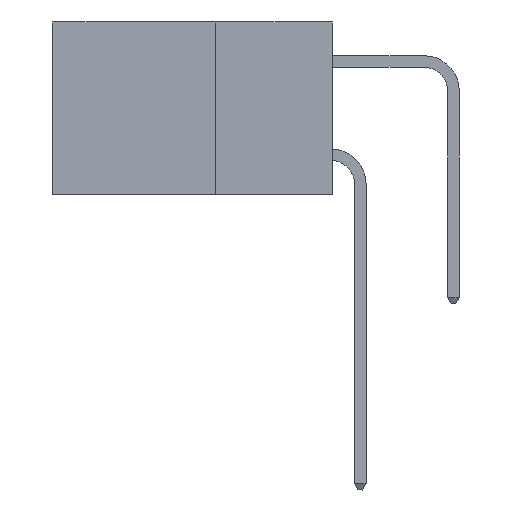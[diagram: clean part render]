
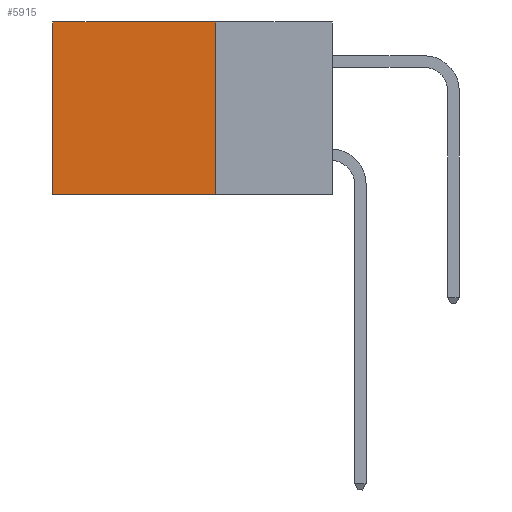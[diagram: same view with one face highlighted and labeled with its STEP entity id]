
A CAD part, left-side view. The second image highlights one B-rep face of the part: STEP entity #5915.
In plain terms, the highlighted planar face has unit normal (-1, 0, 0).
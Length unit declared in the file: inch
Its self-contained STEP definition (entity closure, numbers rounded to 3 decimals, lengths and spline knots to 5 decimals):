
#588 = EDGE_CURVE ( 'NONE', #13878, #1137, #4274, .T. ) ;
#701 = CARTESIAN_POINT ( 'NONE',  ( 0.298, 0.6, 0. ) ) ;
#1094 = EDGE_CURVE ( 'NONE', #13674, #3250, #10222, .T. ) ;
#1137 = VERTEX_POINT ( 'NONE', #9977 ) ;
#1223 = CARTESIAN_POINT ( 'NONE',  ( 0.298, 0.25, 0. ) ) ;
#1358 = DIRECTION ( 'NONE',  ( 0., 1., 0. ) ) ;
#1468 = ORIENTED_EDGE ( 'NONE', *, *, #588, .F. ) ;
#2970 = LINE ( 'NONE', #6909, #15835 ) ;
#3250 = VERTEX_POINT ( 'NONE', #701 ) ;
#3386 = ORIENTED_EDGE ( 'NONE', *, *, #10415, .F. ) ;
#4274 = LINE ( 'NONE', #13102, #8049 ) ;
#4414 = DIRECTION ( 'NONE',  ( 0., 0., -1. ) ) ;
#5915 = ADVANCED_FACE ( 'NONE', ( #8065 ), #13463, .F. ) ;
#5935 = EDGE_CURVE ( 'NONE', #3250, #1137, #11028, .T. ) ;
#6835 = VECTOR ( 'NONE', #1358, 39.37008 ) ;
#6909 = CARTESIAN_POINT ( 'NONE',  ( 0.298, 0.25, 0. ) ) ;
#8049 = VECTOR ( 'NONE', #8203, 39.37008 ) ;
#8065 = FACE_OUTER_BOUND ( 'NONE', #9801, .T. ) ;
#8203 = DIRECTION ( 'NONE',  ( 0., 1., 0. ) ) ;
#9015 = CARTESIAN_POINT ( 'NONE',  ( 0.298, 0.6, 0. ) ) ;
#9801 = EDGE_LOOP ( 'NONE', ( #11238, #1468, #3386, #14372 ) ) ;
#9977 = CARTESIAN_POINT ( 'NONE',  ( 0.298, 0.6, -0.37 ) ) ;
#10222 = LINE ( 'NONE', #1223, #6835 ) ;
#10415 = EDGE_CURVE ( 'NONE', #13674, #13878, #2970, .T. ) ;
#11028 = LINE ( 'NONE', #9015, #13540 ) ;
#11238 = ORIENTED_EDGE ( 'NONE', *, *, #5935, .T. ) ;
#11908 = CARTESIAN_POINT ( 'NONE',  ( 0.298, 0.25, 0. ) ) ;
#12620 = DIRECTION ( 'NONE',  ( 0., 0., -1. ) ) ;
#13102 = CARTESIAN_POINT ( 'NONE',  ( 0.298, 0.25, -0.37 ) ) ;
#13410 = DIRECTION ( 'NONE',  ( 1., 0., 0. ) ) ;
#13443 = CARTESIAN_POINT ( 'NONE',  ( 0.298, 0.25, 0. ) ) ;
#13463 = PLANE ( 'NONE',  #15352 ) ;
#13540 = VECTOR ( 'NONE', #13733, 39.37008 ) ;
#13674 = VERTEX_POINT ( 'NONE', #11908 ) ;
#13733 = DIRECTION ( 'NONE',  ( 0., 0., -1. ) ) ;
#13878 = VERTEX_POINT ( 'NONE', #14675 ) ;
#14372 = ORIENTED_EDGE ( 'NONE', *, *, #1094, .T. ) ;
#14675 = CARTESIAN_POINT ( 'NONE',  ( 0.298, 0.25, -0.37 ) ) ;
#15352 = AXIS2_PLACEMENT_3D ( 'NONE', #13443, #13410, #12620 ) ;
#15835 = VECTOR ( 'NONE', #4414, 39.37008 ) ;
